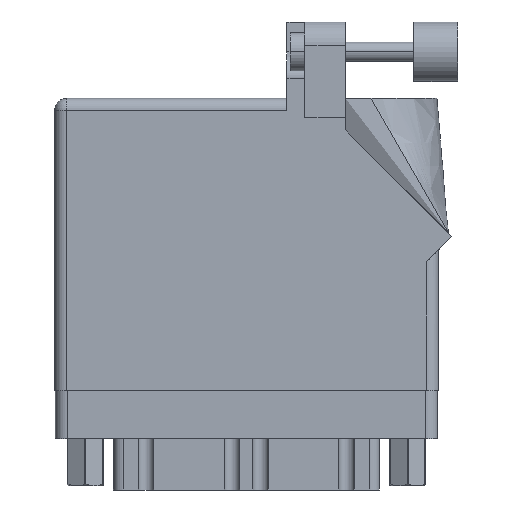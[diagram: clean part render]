
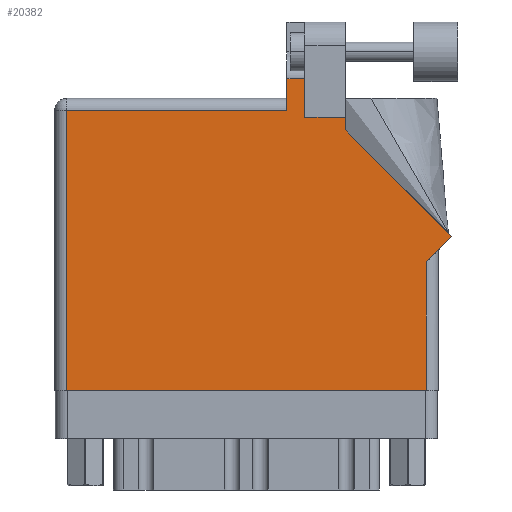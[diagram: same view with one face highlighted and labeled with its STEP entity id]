
A CAD part, front view. The second image highlights one B-rep face of the part: STEP entity #20382.
In plain terms, the highlighted face is planar.
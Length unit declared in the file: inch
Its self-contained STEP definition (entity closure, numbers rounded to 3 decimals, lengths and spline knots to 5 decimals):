
#13 = CARTESIAN_POINT ( 'NONE',  ( 1.524, 1.43, 0. ) ) ;
#3381 = LINE ( 'NONE', #29201, #27855 ) ;
#3386 = LINE ( 'NONE', #39390, #19576 ) ;
#4370 = CARTESIAN_POINT ( 'NONE',  ( 1.311, 1.43, 0. ) ) ;
#4599 = VERTEX_POINT ( 'NONE', #13077 ) ;
#5199 = VECTOR ( 'NONE', #18532, 39.37008 ) ;
#6316 = CARTESIAN_POINT ( 'NONE',  ( 1.524, 1.43, 0. ) ) ;
#6449 = DIRECTION ( 'NONE',  ( 0., 0., -1. ) ) ;
#6452 = DIRECTION ( 'NONE',  ( -1., 0., 0. ) ) ;
#6924 = DIRECTION ( 'NONE',  ( -1., 0., 0. ) ) ;
#7003 = EDGE_CURVE ( 'NONE', #28635, #26983, #19424, .T. ) ;
#7327 = CARTESIAN_POINT ( 'NONE',  ( 0.062, 1.468, 0. ) ) ;
#8147 = CARTESIAN_POINT ( 'NONE',  ( 0., 0., 0. ) ) ;
#8434 = CARTESIAN_POINT ( 'NONE',  ( 1.311, 1.6315, 0. ) ) ;
#9530 = DIRECTION ( 'NONE',  ( 0., 1., 0. ) ) ;
#11397 = ORIENTED_EDGE ( 'NONE', *, *, #7003, .T. ) ;
#11432 = ORIENTED_EDGE ( 'NONE', *, *, #34970, .T. ) ;
#11496 = VECTOR ( 'NONE', #40359, 39.37008 ) ;
#11990 = CARTESIAN_POINT ( 'NONE',  ( 2.08071, 0.80771, 0. ) ) ;
#13077 = CARTESIAN_POINT ( 'NONE',  ( 0.062, 0., 0. ) ) ;
#13170 = EDGE_CURVE ( 'NONE', #18253, #18500, #40618, .T. ) ;
#13752 = CARTESIAN_POINT ( 'NONE',  ( 0., 1.468, 0. ) ) ;
#13969 = LINE ( 'NONE', #18055, #5199 ) ;
#14750 = EDGE_CURVE ( 'NONE', #26983, #29735, #13969, .T. ) ;
#15485 = CARTESIAN_POINT ( 'NONE',  ( 1.948, 0.675, 0. ) ) ;
#15849 = DIRECTION ( 'NONE',  ( 1., 0., 0. ) ) ;
#15863 = EDGE_CURVE ( 'NONE', #23487, #43925, #24099, .T. ) ;
#16515 = ORIENTED_EDGE ( 'NONE', *, *, #40974, .T. ) ;
#17601 = LINE ( 'NONE', #13752, #27288 ) ;
#17671 = ORIENTED_EDGE ( 'NONE', *, *, #20467, .T. ) ;
#17984 = CARTESIAN_POINT ( 'NONE',  ( 1.217, 1.6315, 0. ) ) ;
#18055 = CARTESIAN_POINT ( 'NONE',  ( 2.01, 0.737, 0. ) ) ;
#18253 = VERTEX_POINT ( 'NONE', #6316 ) ;
#18446 = CARTESIAN_POINT ( 'NONE',  ( 0.062, 0., 0. ) ) ;
#18500 = VERTEX_POINT ( 'NONE', #4370 ) ;
#18532 = DIRECTION ( 'NONE',  ( 0.707, 0.707, 0. ) ) ;
#18735 = VECTOR ( 'NONE', #15849, 39.37008 ) ;
#19214 = DIRECTION ( 'NONE',  ( -0.707, 0.707, 0. ) ) ;
#19424 = LINE ( 'NONE', #27412, #25144 ) ;
#19576 = VECTOR ( 'NONE', #31876, 39.37008 ) ;
#19636 = AXIS2_PLACEMENT_3D ( 'NONE', #46824, #6449, #6924 ) ;
#20382 = ADVANCED_FACE ( 'NONE', ( #21405 ), #39809, .F. ) ;
#20467 = EDGE_CURVE ( 'NONE', #29735, #22973, #22151, .T. ) ;
#20650 = ORIENTED_EDGE ( 'NONE', *, *, #43580, .T. ) ;
#20685 = VERTEX_POINT ( 'NONE', #23818 ) ;
#20693 = CARTESIAN_POINT ( 'NONE',  ( 1.64177, 1.6315, 0. ) ) ;
#20757 = DIRECTION ( 'NONE',  ( -1., 0., 0. ) ) ;
#21214 = CARTESIAN_POINT ( 'NONE',  ( 2.08071, 0.80771, 0. ) ) ;
#21405 = FACE_OUTER_BOUND ( 'NONE', #35775, .T. ) ;
#22151 = LINE ( 'NONE', #11990, #29709 ) ;
#22973 = VERTEX_POINT ( 'NONE', #33140 ) ;
#23487 = VERTEX_POINT ( 'NONE', #8434 ) ;
#23818 = CARTESIAN_POINT ( 'NONE',  ( 1.217, 1.468, 0. ) ) ;
#24046 = ORIENTED_EDGE ( 'NONE', *, *, #14750, .T. ) ;
#24099 = LINE ( 'NONE', #20693, #25612 ) ;
#24302 = VERTEX_POINT ( 'NONE', #7327 ) ;
#24912 = DIRECTION ( 'NONE',  ( 0., 1., 0. ) ) ;
#25144 = VECTOR ( 'NONE', #9530, 39.37008 ) ;
#25568 = DIRECTION ( 'NONE',  ( 0., -1., 0. ) ) ;
#25612 = VECTOR ( 'NONE', #6452, 39.37008 ) ;
#26199 = LINE ( 'NONE', #18446, #46555 ) ;
#26983 = VERTEX_POINT ( 'NONE', #15485 ) ;
#27288 = VECTOR ( 'NONE', #20757, 39.37008 ) ;
#27412 = CARTESIAN_POINT ( 'NONE',  ( 1.948, 0.737, 0. ) ) ;
#27855 = VECTOR ( 'NONE', #25568, 39.37008 ) ;
#28635 = VERTEX_POINT ( 'NONE', #44731 ) ;
#28764 = LINE ( 'NONE', #46440, #32647 ) ;
#28907 = EDGE_CURVE ( 'NONE', #20685, #24302, #17601, .T. ) ;
#28927 = EDGE_CURVE ( 'NONE', #22973, #18253, #3386, .T. ) ;
#29201 = CARTESIAN_POINT ( 'NONE',  ( 1.217, 1.53, 0. ) ) ;
#29709 = VECTOR ( 'NONE', #19214, 39.37008 ) ;
#29735 = VERTEX_POINT ( 'NONE', #21214 ) ;
#31746 = ORIENTED_EDGE ( 'NONE', *, *, #40226, .T. ) ;
#31876 = DIRECTION ( 'NONE',  ( 0., 1., 0. ) ) ;
#32647 = VECTOR ( 'NONE', #24912, 39.37008 ) ;
#33140 = CARTESIAN_POINT ( 'NONE',  ( 1.524, 1.36442, 0. ) ) ;
#34478 = LINE ( 'NONE', #8147, #18735 ) ;
#34970 = EDGE_CURVE ( 'NONE', #43925, #20685, #3381, .T. ) ;
#35775 = EDGE_LOOP ( 'NONE', ( #16515, #36824, #11432, #47136, #31746, #20650, #11397, #24046, #17671, #45459, #43763 ) ) ;
#36824 = ORIENTED_EDGE ( 'NONE', *, *, #15863, .T. ) ;
#39390 = CARTESIAN_POINT ( 'NONE',  ( 1.524, 1.36442, 0. ) ) ;
#39809 = PLANE ( 'NONE',  #19636 ) ;
#40226 = EDGE_CURVE ( 'NONE', #24302, #4599, #26199, .T. ) ;
#40359 = DIRECTION ( 'NONE',  ( -1., 0., 0. ) ) ;
#40618 = LINE ( 'NONE', #13, #11496 ) ;
#40956 = DIRECTION ( 'NONE',  ( 0., -1., 0. ) ) ;
#40974 = EDGE_CURVE ( 'NONE', #18500, #23487, #28764, .T. ) ;
#43580 = EDGE_CURVE ( 'NONE', #4599, #28635, #34478, .T. ) ;
#43763 = ORIENTED_EDGE ( 'NONE', *, *, #13170, .T. ) ;
#43925 = VERTEX_POINT ( 'NONE', #17984 ) ;
#44731 = CARTESIAN_POINT ( 'NONE',  ( 1.948, 0., 0. ) ) ;
#45459 = ORIENTED_EDGE ( 'NONE', *, *, #28927, .T. ) ;
#46440 = CARTESIAN_POINT ( 'NONE',  ( 1.311, 1.43, 0. ) ) ;
#46555 = VECTOR ( 'NONE', #40956, 39.37008 ) ;
#46824 = CARTESIAN_POINT ( 'NONE',  ( 0., 1.53, 0. ) ) ;
#47136 = ORIENTED_EDGE ( 'NONE', *, *, #28907, .T. ) ;
